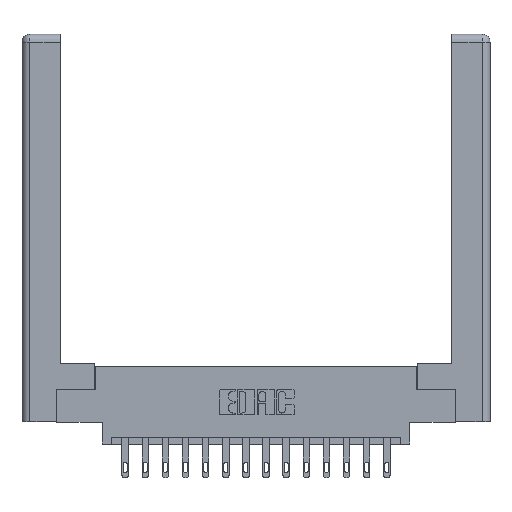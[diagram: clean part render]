
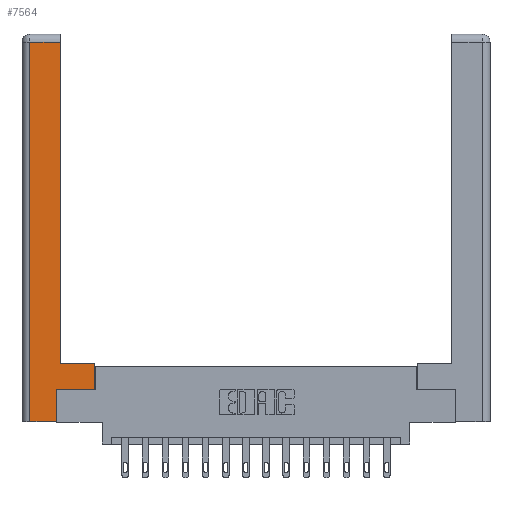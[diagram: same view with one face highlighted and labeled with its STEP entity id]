
A CAD part, top view. The second image highlights one B-rep face of the part: STEP entity #7564.
In plain terms, the highlighted planar face has unit normal (0, 0, 1).
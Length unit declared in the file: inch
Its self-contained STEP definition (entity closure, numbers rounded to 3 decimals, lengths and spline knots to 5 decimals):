
#783 = DIRECTION ( 'NONE',  ( -1., 0., 0. ) ) ;
#857 = CARTESIAN_POINT ( 'NONE',  ( 0.565, 0.45, 0. ) ) ;
#1095 = EDGE_CURVE ( 'NONE', #7017, #11145, #13843, .T. ) ;
#1124 = ORIENTED_EDGE ( 'NONE', *, *, #9004, .T. ) ;
#1828 = CARTESIAN_POINT ( 'NONE',  ( 0.295, 2.94, 0. ) ) ;
#1861 = VERTEX_POINT ( 'NONE', #15703 ) ;
#2169 = EDGE_CURVE ( 'NONE', #11065, #10239, #16947, .T. ) ;
#2625 = ORIENTED_EDGE ( 'NONE', *, *, #13088, .T. ) ;
#2644 = DIRECTION ( 'NONE',  ( -1., 0., 0. ) ) ;
#3031 = ORIENTED_EDGE ( 'NONE', *, *, #1095, .T. ) ;
#3098 = LINE ( 'NONE', #11108, #8944 ) ;
#3108 = DIRECTION ( 'NONE',  ( 0., 1., 0. ) ) ;
#3222 = FACE_OUTER_BOUND ( 'NONE', #3352, .T. ) ;
#3265 = AXIS2_PLACEMENT_3D ( 'NONE', #8769, #3406, #783 ) ;
#3282 = VECTOR ( 'NONE', #2644, 39.37008 ) ;
#3352 = EDGE_LOOP ( 'NONE', ( #11539, #2625, #15155, #3031, #3812, #1124, #16324, #5781 ) ) ;
#3406 = DIRECTION ( 'NONE',  ( 0., 0., -1. ) ) ;
#3489 = DIRECTION ( 'NONE',  ( 1., 0., 0. ) ) ;
#3812 = ORIENTED_EDGE ( 'NONE', *, *, #15777, .T. ) ;
#4193 = LINE ( 'NONE', #10143, #12098 ) ;
#4314 = CARTESIAN_POINT ( 'NONE',  ( 0.565, 0.45, 0. ) ) ;
#4692 = CARTESIAN_POINT ( 'NONE',  ( 0.295, 0.45, 0. ) ) ;
#4773 = EDGE_CURVE ( 'NONE', #12589, #5176, #3098, .T. ) ;
#5176 = VERTEX_POINT ( 'NONE', #1828 ) ;
#5304 = EDGE_CURVE ( 'NONE', #10239, #12589, #13686, .T. ) ;
#5781 = ORIENTED_EDGE ( 'NONE', *, *, #5304, .T. ) ;
#6352 = DIRECTION ( 'NONE',  ( 1., 0., 0. ) ) ;
#6497 = VECTOR ( 'NONE', #3108, 39.37008 ) ;
#7017 = VERTEX_POINT ( 'NONE', #7409 ) ;
#7362 = CARTESIAN_POINT ( 'NONE',  ( 0.265, 0., 0. ) ) ;
#7409 = CARTESIAN_POINT ( 'NONE',  ( 0.0615, 0., 0. ) ) ;
#7564 = ADVANCED_FACE ( 'NONE', ( #3222 ), #8601, .F. ) ;
#7870 = CARTESIAN_POINT ( 'NONE',  ( 0.295, 0.45, 0. ) ) ;
#8601 = PLANE ( 'NONE',  #3265 ) ;
#8769 = CARTESIAN_POINT ( 'NONE',  ( 0., 0., 0. ) ) ;
#8865 = DIRECTION ( 'NONE',  ( -1., 0., 0. ) ) ;
#8944 = VECTOR ( 'NONE', #11628, 39.37008 ) ;
#9004 = EDGE_CURVE ( 'NONE', #1861, #11065, #17076, .T. ) ;
#9223 = CARTESIAN_POINT ( 'NONE',  ( 0.265, 0., 0. ) ) ;
#9642 = CARTESIAN_POINT ( 'NONE',  ( 0.265, 0.245, 0. ) ) ;
#10065 = CARTESIAN_POINT ( 'NONE',  ( 0.565, 0.245, 0. ) ) ;
#10143 = CARTESIAN_POINT ( 'NONE',  ( 0.0615, 0., 0. ) ) ;
#10181 = EDGE_CURVE ( 'NONE', #17157, #7017, #4193, .T. ) ;
#10239 = VERTEX_POINT ( 'NONE', #4314 ) ;
#10419 = CARTESIAN_POINT ( 'NONE',  ( 0.0615, 2.94, 0. ) ) ;
#10624 = DIRECTION ( 'NONE',  ( 0., 1., 0. ) ) ;
#10652 = LINE ( 'NONE', #9642, #6497 ) ;
#11065 = VERTEX_POINT ( 'NONE', #15248 ) ;
#11108 = CARTESIAN_POINT ( 'NONE',  ( 0.295, 3., 0. ) ) ;
#11145 = VERTEX_POINT ( 'NONE', #7362 ) ;
#11539 = ORIENTED_EDGE ( 'NONE', *, *, #4773, .T. ) ;
#11628 = DIRECTION ( 'NONE',  ( 0., 1., 0. ) ) ;
#12040 = LINE ( 'NONE', #13220, #3282 ) ;
#12098 = VECTOR ( 'NONE', #12877, 39.37008 ) ;
#12589 = VERTEX_POINT ( 'NONE', #7870 ) ;
#12606 = VECTOR ( 'NONE', #10624, 39.37008 ) ;
#12877 = DIRECTION ( 'NONE',  ( 0., -1., 0. ) ) ;
#13088 = EDGE_CURVE ( 'NONE', #5176, #17157, #12040, .T. ) ;
#13220 = CARTESIAN_POINT ( 'NONE',  ( 0.0615, 2.94, 0. ) ) ;
#13338 = VECTOR ( 'NONE', #3489, 39.37008 ) ;
#13686 = LINE ( 'NONE', #4692, #13884 ) ;
#13843 = LINE ( 'NONE', #9223, #16564 ) ;
#13884 = VECTOR ( 'NONE', #8865, 39.37008 ) ;
#15155 = ORIENTED_EDGE ( 'NONE', *, *, #10181, .T. ) ;
#15248 = CARTESIAN_POINT ( 'NONE',  ( 0.565, 0.245, 0. ) ) ;
#15703 = CARTESIAN_POINT ( 'NONE',  ( 0.265, 0.245, 0. ) ) ;
#15777 = EDGE_CURVE ( 'NONE', #11145, #1861, #10652, .T. ) ;
#16324 = ORIENTED_EDGE ( 'NONE', *, *, #2169, .T. ) ;
#16564 = VECTOR ( 'NONE', #6352, 39.37008 ) ;
#16947 = LINE ( 'NONE', #857, #12606 ) ;
#17076 = LINE ( 'NONE', #10065, #13338 ) ;
#17157 = VERTEX_POINT ( 'NONE', #10419 ) ;
